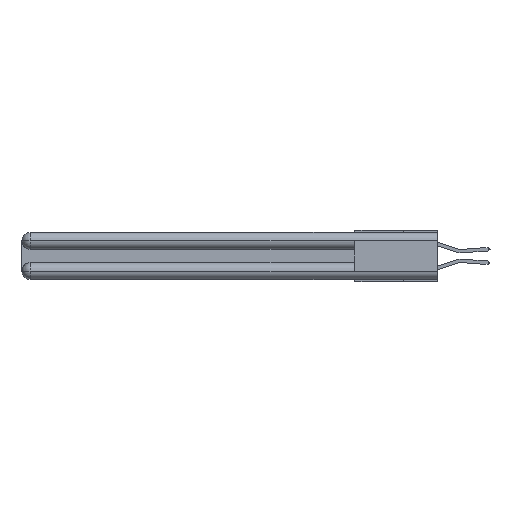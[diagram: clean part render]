
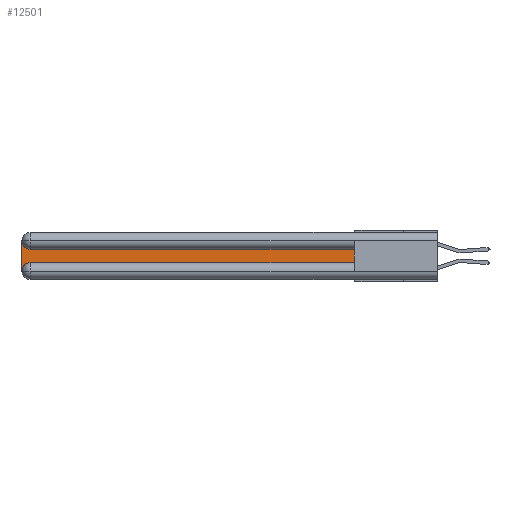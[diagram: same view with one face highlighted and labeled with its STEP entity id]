
A CAD part, left-side view. The second image highlights one B-rep face of the part: STEP entity #12501.
In plain terms, the highlighted planar face has unit normal (-1, 0, 0).
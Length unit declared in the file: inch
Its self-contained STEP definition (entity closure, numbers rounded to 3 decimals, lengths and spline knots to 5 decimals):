
#385 = DIRECTION ( 'NONE',  ( 0., 0., -1. ) ) ;
#754 = CIRCLE ( 'NONE', #30116, 0.06 ) ;
#2651 = CARTESIAN_POINT ( 'NONE',  ( 0.075, 2.94, -0.2175 ) ) ;
#2807 = CARTESIAN_POINT ( 'NONE',  ( 0.075, 3., -0.1225 ) ) ;
#3583 = CARTESIAN_POINT ( 'NONE',  ( 0.075, 2.94, -0.2775 ) ) ;
#3649 = FACE_OUTER_BOUND ( 'NONE', #12845, .T. ) ;
#4594 = CARTESIAN_POINT ( 'NONE',  ( 0.075, 3., -0.2775 ) ) ;
#5348 = DIRECTION ( 'NONE',  ( 1., 0., 0. ) ) ;
#5792 = VECTOR ( 'NONE', #15169, 39.37008 ) ;
#7095 = CARTESIAN_POINT ( 'NONE',  ( 0.075, 2.94, -0.1225 ) ) ;
#7186 = ORIENTED_EDGE ( 'NONE', *, *, #9281, .T. ) ;
#7867 = ORIENTED_EDGE ( 'NONE', *, *, #10838, .T. ) ;
#7871 = VECTOR ( 'NONE', #16824, 39.37008 ) ;
#8200 = EDGE_CURVE ( 'NONE', #14026, #31071, #18897, .T. ) ;
#8319 = CARTESIAN_POINT ( 'NONE',  ( 0.075, 0.6, -0.1225 ) ) ;
#8951 = DIRECTION ( 'NONE',  ( 1., 0., 0. ) ) ;
#8994 = CARTESIAN_POINT ( 'NONE',  ( 0.075, 2.94, -0.0625 ) ) ;
#9281 = EDGE_CURVE ( 'NONE', #15609, #16546, #754, .T. ) ;
#10583 = CARTESIAN_POINT ( 'NONE',  ( 0.075, 3., -0.0625 ) ) ;
#10838 = EDGE_CURVE ( 'NONE', #20402, #14026, #24317, .T. ) ;
#11642 = DIRECTION ( 'NONE',  ( 1., 0., 0. ) ) ;
#12205 = ORIENTED_EDGE ( 'NONE', *, *, #31905, .T. ) ;
#12501 = ADVANCED_FACE ( 'NONE', ( #3649 ), #15775, .F. ) ;
#12845 = EDGE_LOOP ( 'NONE', ( #18332, #14683, #12205, #7186, #15846, #7867 ) ) ;
#13557 = EDGE_CURVE ( 'NONE', #31071, #23808, #24751, .T. ) ;
#14026 = VERTEX_POINT ( 'NONE', #8319 ) ;
#14391 = DIRECTION ( 'NONE',  ( 0., 0., -1. ) ) ;
#14403 = CARTESIAN_POINT ( 'NONE',  ( 0.075, 3., -0.2175 ) ) ;
#14683 = ORIENTED_EDGE ( 'NONE', *, *, #13557, .T. ) ;
#15169 = DIRECTION ( 'NONE',  ( 0., 1., 0. ) ) ;
#15609 = VERTEX_POINT ( 'NONE', #4594 ) ;
#15775 = PLANE ( 'NONE',  #26000 ) ;
#15846 = ORIENTED_EDGE ( 'NONE', *, *, #16726, .T. ) ;
#16546 = VERTEX_POINT ( 'NONE', #2651 ) ;
#16726 = EDGE_CURVE ( 'NONE', #16546, #20402, #24968, .T. ) ;
#16777 = DIRECTION ( 'NONE',  ( 0., -1., 0. ) ) ;
#16824 = DIRECTION ( 'NONE',  ( 0., 0., 1. ) ) ;
#18332 = ORIENTED_EDGE ( 'NONE', *, *, #8200, .T. ) ;
#18897 = LINE ( 'NONE', #20556, #5792 ) ;
#19634 = VECTOR ( 'NONE', #27359, 39.37008 ) ;
#20402 = VERTEX_POINT ( 'NONE', #29686 ) ;
#20556 = CARTESIAN_POINT ( 'NONE',  ( 0.075, 0.6, -0.1225 ) ) ;
#21561 = DIRECTION ( 'NONE',  ( 0., 0., -1. ) ) ;
#21671 = LINE ( 'NONE', #14403, #19634 ) ;
#22058 = CARTESIAN_POINT ( 'NONE',  ( 0.075, 0.6, -0.2175 ) ) ;
#22487 = VECTOR ( 'NONE', #16777, 39.37008 ) ;
#23808 = VERTEX_POINT ( 'NONE', #10583 ) ;
#24317 = LINE ( 'NONE', #22058, #7871 ) ;
#24751 = CIRCLE ( 'NONE', #29321, 0.06 ) ;
#24968 = LINE ( 'NONE', #32478, #22487 ) ;
#26000 = AXIS2_PLACEMENT_3D ( 'NONE', #2807, #5348, #385 ) ;
#27359 = DIRECTION ( 'NONE',  ( 0., 0., -1. ) ) ;
#29321 = AXIS2_PLACEMENT_3D ( 'NONE', #8994, #11642, #14391 ) ;
#29686 = CARTESIAN_POINT ( 'NONE',  ( 0.075, 0.6, -0.2175 ) ) ;
#30116 = AXIS2_PLACEMENT_3D ( 'NONE', #3583, #8951, #21561 ) ;
#31071 = VERTEX_POINT ( 'NONE', #7095 ) ;
#31905 = EDGE_CURVE ( 'NONE', #23808, #15609, #21671, .T. ) ;
#32478 = CARTESIAN_POINT ( 'NONE',  ( 0.075, 0.6, -0.2175 ) ) ;
